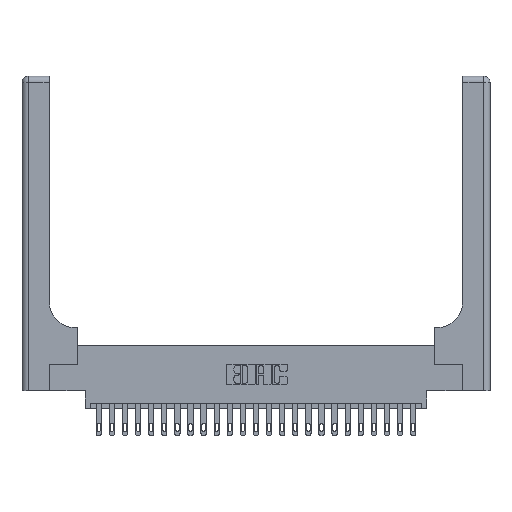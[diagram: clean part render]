
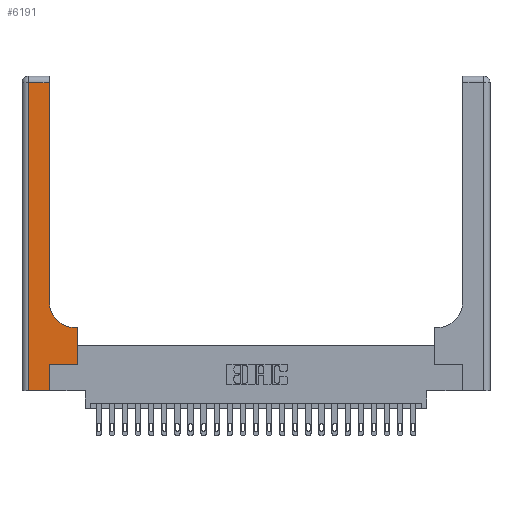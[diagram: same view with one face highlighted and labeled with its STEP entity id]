
A CAD part, top view. The second image highlights one B-rep face of the part: STEP entity #6191.
In plain terms, the highlighted planar face has unit normal (0, 0, 1).
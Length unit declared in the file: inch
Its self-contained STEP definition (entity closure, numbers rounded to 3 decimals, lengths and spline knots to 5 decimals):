
#427 = PLANE ( 'NONE',  #23444 ) ;
#936 = VERTEX_POINT ( 'NONE', #23625 ) ;
#1240 = VERTEX_POINT ( 'NONE', #9955 ) ;
#1335 = ORIENTED_EDGE ( 'NONE', *, *, #19737, .T. ) ;
#1347 = ORIENTED_EDGE ( 'NONE', *, *, #7663, .T. ) ;
#1363 = DIRECTION ( 'NONE',  ( -1., 0., 0. ) ) ;
#1856 = LINE ( 'NONE', #24126, #6697 ) ;
#2144 = CARTESIAN_POINT ( 'NONE',  ( 0.06, 3., 0.37 ) ) ;
#2899 = ORIENTED_EDGE ( 'NONE', *, *, #19192, .T. ) ;
#3433 = VECTOR ( 'NONE', #15968, 39.37008 ) ;
#3469 = VERTEX_POINT ( 'NONE', #23865 ) ;
#3642 = DIRECTION ( 'NONE',  ( 0., 1., 0. ) ) ;
#4126 = VERTEX_POINT ( 'NONE', #12385 ) ;
#4171 = LINE ( 'NONE', #9830, #14407 ) ;
#4230 = CARTESIAN_POINT ( 'NONE',  ( 0., 3., 0.37 ) ) ;
#4292 = VERTEX_POINT ( 'NONE', #16882 ) ;
#4443 = EDGE_CURVE ( 'NONE', #936, #4292, #8040, .T. ) ;
#5111 = CARTESIAN_POINT ( 'NONE',  ( 0., 0., 0.37 ) ) ;
#5405 = AXIS2_PLACEMENT_3D ( 'NONE', #7932, #21066, #18859 ) ;
#5454 = CARTESIAN_POINT ( 'NONE',  ( 0.265, 0., 0.37 ) ) ;
#5507 = VECTOR ( 'NONE', #12621, 39.37008 ) ;
#5726 = VERTEX_POINT ( 'NONE', #17299 ) ;
#6191 = ADVANCED_FACE ( 'NONE', ( #17506 ), #427, .F. ) ;
#6606 = EDGE_CURVE ( 'NONE', #1240, #5726, #4171, .T. ) ;
#6697 = VECTOR ( 'NONE', #22413, 39.37008 ) ;
#7302 = LINE ( 'NONE', #5454, #18991 ) ;
#7663 = EDGE_CURVE ( 'NONE', #4292, #12301, #23763, .T. ) ;
#7932 = CARTESIAN_POINT ( 'NONE',  ( 0.51, 0.85, 0.37 ) ) ;
#8040 = LINE ( 'NONE', #17257, #22976 ) ;
#8162 = VECTOR ( 'NONE', #1363, 39.37008 ) ;
#8193 = CARTESIAN_POINT ( 'NONE',  ( 0.265, 0.25, 0.37 ) ) ;
#8360 = EDGE_LOOP ( 'NONE', ( #21653, #2899, #14223, #10016, #14564, #1335, #19138, #1347, #20796 ) ) ;
#9338 = VECTOR ( 'NONE', #22550, 39.37008 ) ;
#9830 = CARTESIAN_POINT ( 'NONE',  ( 0.26, 3., 0.37 ) ) ;
#9955 = CARTESIAN_POINT ( 'NONE',  ( 0.26, 0.85, 0.37 ) ) ;
#9992 = EDGE_CURVE ( 'NONE', #12118, #3469, #11633, .T. ) ;
#10016 = ORIENTED_EDGE ( 'NONE', *, *, #13555, .T. ) ;
#10022 = EDGE_CURVE ( 'NONE', #12301, #1240, #23503, .T. ) ;
#11577 = CARTESIAN_POINT ( 'NONE',  ( 0.06, 2.94, 0.37 ) ) ;
#11633 = LINE ( 'NONE', #2144, #9338 ) ;
#12118 = VERTEX_POINT ( 'NONE', #11577 ) ;
#12301 = VERTEX_POINT ( 'NONE', #17934 ) ;
#12385 = CARTESIAN_POINT ( 'NONE',  ( 0.265, 0., 0.37 ) ) ;
#12621 = DIRECTION ( 'NONE',  ( -1., 0., 0. ) ) ;
#13555 = EDGE_CURVE ( 'NONE', #3469, #4126, #18158, .T. ) ;
#13700 = DIRECTION ( 'NONE',  ( 0., 0., -1. ) ) ;
#14223 = ORIENTED_EDGE ( 'NONE', *, *, #9992, .T. ) ;
#14407 = VECTOR ( 'NONE', #15485, 39.37008 ) ;
#14564 = ORIENTED_EDGE ( 'NONE', *, *, #22491, .T. ) ;
#14700 = LINE ( 'NONE', #21948, #5507 ) ;
#15148 = VERTEX_POINT ( 'NONE', #8193 ) ;
#15485 = DIRECTION ( 'NONE',  ( 0., 1., 0. ) ) ;
#15968 = DIRECTION ( 'NONE',  ( 1., 0., 0. ) ) ;
#16882 = CARTESIAN_POINT ( 'NONE',  ( 0.528, 0.6, 0.37 ) ) ;
#17257 = CARTESIAN_POINT ( 'NONE',  ( 0.528, 0.25, 0.37 ) ) ;
#17299 = CARTESIAN_POINT ( 'NONE',  ( 0.26, 2.94, 0.37 ) ) ;
#17506 = FACE_OUTER_BOUND ( 'NONE', #8360, .T. ) ;
#17934 = CARTESIAN_POINT ( 'NONE',  ( 0.51, 0.6, 0.37 ) ) ;
#17971 = CARTESIAN_POINT ( 'NONE',  ( 0.26, 0.6, 0.37 ) ) ;
#18158 = LINE ( 'NONE', #5111, #3433 ) ;
#18859 = DIRECTION ( 'NONE',  ( 1., 0., 0. ) ) ;
#18991 = VECTOR ( 'NONE', #3642, 39.37008 ) ;
#19138 = ORIENTED_EDGE ( 'NONE', *, *, #4443, .T. ) ;
#19192 = EDGE_CURVE ( 'NONE', #5726, #12118, #14700, .T. ) ;
#19737 = EDGE_CURVE ( 'NONE', #15148, #936, #1856, .T. ) ;
#20796 = ORIENTED_EDGE ( 'NONE', *, *, #10022, .T. ) ;
#21055 = DIRECTION ( 'NONE',  ( 0., 1., 0. ) ) ;
#21066 = DIRECTION ( 'NONE',  ( 0., 0., -1. ) ) ;
#21653 = ORIENTED_EDGE ( 'NONE', *, *, #6606, .T. ) ;
#21948 = CARTESIAN_POINT ( 'NONE',  ( 0., 2.94, 0.37 ) ) ;
#22413 = DIRECTION ( 'NONE',  ( 1., 0., 0. ) ) ;
#22491 = EDGE_CURVE ( 'NONE', #4126, #15148, #7302, .T. ) ;
#22550 = DIRECTION ( 'NONE',  ( 0., -1., 0. ) ) ;
#22976 = VECTOR ( 'NONE', #21055, 39.37008 ) ;
#23177 = DIRECTION ( 'NONE',  ( -1., 0., 0. ) ) ;
#23444 = AXIS2_PLACEMENT_3D ( 'NONE', #4230, #13700, #23177 ) ;
#23503 = CIRCLE ( 'NONE', #5405, 0.25 ) ;
#23625 = CARTESIAN_POINT ( 'NONE',  ( 0.528, 0.25, 0.37 ) ) ;
#23763 = LINE ( 'NONE', #17971, #8162 ) ;
#23865 = CARTESIAN_POINT ( 'NONE',  ( 0.06, 0., 0.37 ) ) ;
#24126 = CARTESIAN_POINT ( 'NONE',  ( 0.265, 0.25, 0.37 ) ) ;
